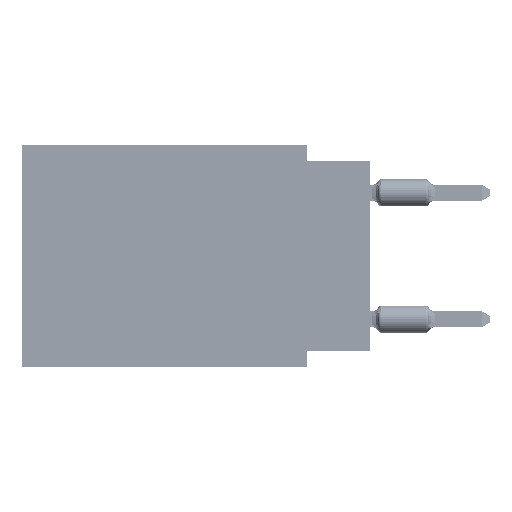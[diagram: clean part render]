
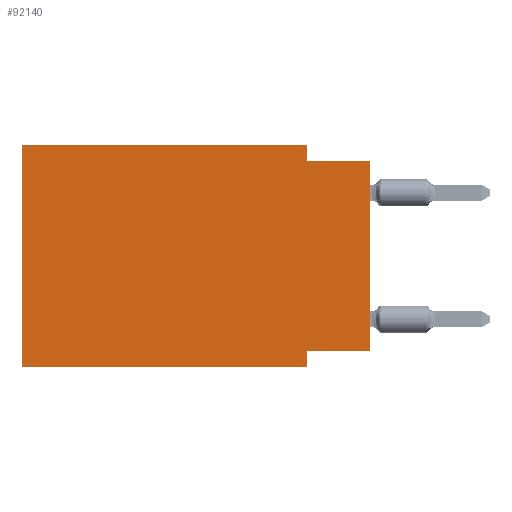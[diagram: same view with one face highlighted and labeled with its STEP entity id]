
A CAD part, left-side view. The second image highlights one B-rep face of the part: STEP entity #92140.
In plain terms, the highlighted planar face has unit normal (-1, 0, 0).
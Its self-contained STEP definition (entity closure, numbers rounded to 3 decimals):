
#493 = CARTESIAN_POINT ( 'NONE',  ( 0., 2.54, -8.89 ) ) ;
#1888 = CARTESIAN_POINT ( 'NONE',  ( 0., 13.97, 0. ) ) ;
#4435 = VECTOR ( 'NONE', #46885, 1000. ) ;
#5771 = VECTOR ( 'NONE', #45051, 1000. ) ;
#9405 = LINE ( 'NONE', #62555, #5771 ) ;
#11519 = CARTESIAN_POINT ( 'NONE',  ( 0., 0., -0.635 ) ) ;
#13031 = LINE ( 'NONE', #111192, #33113 ) ;
#13939 = VERTEX_POINT ( 'NONE', #55279 ) ;
#15241 = CARTESIAN_POINT ( 'NONE',  ( 0., 0., -0.635 ) ) ;
#15337 = FACE_OUTER_BOUND ( 'NONE', #18035, .T. ) ;
#15803 = LINE ( 'NONE', #51438, #30548 ) ;
#17249 = DIRECTION ( 'NONE',  ( 0., 0., -1. ) ) ;
#17670 = EDGE_CURVE ( 'NONE', #100016, #37350, #30232, .T. ) ;
#17733 = ORIENTED_EDGE ( 'NONE', *, *, #40142, .T. ) ;
#18035 = EDGE_LOOP ( 'NONE', ( #17733, #66285, #18633, #58168, #27498, #62420, #31094, #110468 ) ) ;
#18633 = ORIENTED_EDGE ( 'NONE', *, *, #108957, .F. ) ;
#22695 = VECTOR ( 'NONE', #17249, 1000. ) ;
#27498 = ORIENTED_EDGE ( 'NONE', *, *, #30764, .F. ) ;
#27574 = CARTESIAN_POINT ( 'NONE',  ( 0., 13.97, -8.89 ) ) ;
#29958 = CARTESIAN_POINT ( 'NONE',  ( 0., 2.54, -0.635 ) ) ;
#30232 = LINE ( 'NONE', #37839, #78064 ) ;
#30548 = VECTOR ( 'NONE', #78305, 1000. ) ;
#30764 = EDGE_CURVE ( 'NONE', #100016, #57945, #81920, .T. ) ;
#31094 = ORIENTED_EDGE ( 'NONE', *, *, #78271, .F. ) ;
#32855 = DIRECTION ( 'NONE',  ( 1., 0., 0. ) ) ;
#33113 = VECTOR ( 'NONE', #48692, 1000. ) ;
#35313 = VERTEX_POINT ( 'NONE', #29958 ) ;
#35346 = LINE ( 'NONE', #72120, #22695 ) ;
#37350 = VERTEX_POINT ( 'NONE', #493 ) ;
#37826 = DIRECTION ( 'NONE',  ( 0., 1., 0. ) ) ;
#37839 = CARTESIAN_POINT ( 'NONE',  ( 0., 13.97, -8.89 ) ) ;
#38108 = AXIS2_PLACEMENT_3D ( 'NONE', #61469, #32855, #42779 ) ;
#38359 = VERTEX_POINT ( 'NONE', #48074 ) ;
#40142 = EDGE_CURVE ( 'NONE', #38359, #90475, #13031, .T. ) ;
#41632 = PLANE ( 'NONE',  #38108 ) ;
#42779 = DIRECTION ( 'NONE',  ( 0., 0., -1. ) ) ;
#45051 = DIRECTION ( 'NONE',  ( 0., 0., -1. ) ) ;
#46885 = DIRECTION ( 'NONE',  ( 0., 0., 1. ) ) ;
#48074 = CARTESIAN_POINT ( 'NONE',  ( 0., 0., -8.255 ) ) ;
#48692 = DIRECTION ( 'NONE',  ( 0., 0., 1. ) ) ;
#51438 = CARTESIAN_POINT ( 'NONE',  ( 0., 13.97, 0. ) ) ;
#55279 = CARTESIAN_POINT ( 'NONE',  ( 0., 2.54, -8.255 ) ) ;
#55934 = DIRECTION ( 'NONE',  ( 0., -1., 0. ) ) ;
#56464 = EDGE_CURVE ( 'NONE', #57945, #102134, #15803, .T. ) ;
#57202 = CARTESIAN_POINT ( 'NONE',  ( 0., 13.97, 0. ) ) ;
#57323 = VECTOR ( 'NONE', #37826, 1000. ) ;
#57945 = VERTEX_POINT ( 'NONE', #57202 ) ;
#58168 = ORIENTED_EDGE ( 'NONE', *, *, #56464, .F. ) ;
#61469 = CARTESIAN_POINT ( 'NONE',  ( 0., 13.97, 0. ) ) ;
#62420 = ORIENTED_EDGE ( 'NONE', *, *, #17670, .T. ) ;
#62555 = CARTESIAN_POINT ( 'NONE',  ( 0., 2.54, -8.89 ) ) ;
#66285 = ORIENTED_EDGE ( 'NONE', *, *, #69022, .F. ) ;
#69022 = EDGE_CURVE ( 'NONE', #35313, #90475, #91560, .T. ) ;
#72120 = CARTESIAN_POINT ( 'NONE',  ( 0., 2.54, 0. ) ) ;
#73452 = CARTESIAN_POINT ( 'NONE',  ( 0., 0., -8.255 ) ) ;
#78064 = VECTOR ( 'NONE', #55934, 1000. ) ;
#78271 = EDGE_CURVE ( 'NONE', #13939, #37350, #9405, .T. ) ;
#78305 = DIRECTION ( 'NONE',  ( 0., -1., 0. ) ) ;
#81625 = LINE ( 'NONE', #73452, #57323 ) ;
#81920 = LINE ( 'NONE', #1888, #4435 ) ;
#82784 = DIRECTION ( 'NONE',  ( 0., -1., 0. ) ) ;
#90475 = VERTEX_POINT ( 'NONE', #15241 ) ;
#91560 = LINE ( 'NONE', #11519, #96959 ) ;
#92140 = ADVANCED_FACE ( 'NONE', ( #15337 ), #41632, .F. ) ;
#93863 = CARTESIAN_POINT ( 'NONE',  ( 0., 2.54, 0. ) ) ;
#96959 = VECTOR ( 'NONE', #82784, 1000. ) ;
#100016 = VERTEX_POINT ( 'NONE', #27574 ) ;
#102041 = EDGE_CURVE ( 'NONE', #38359, #13939, #81625, .T. ) ;
#102134 = VERTEX_POINT ( 'NONE', #93863 ) ;
#108957 = EDGE_CURVE ( 'NONE', #102134, #35313, #35346, .T. ) ;
#110468 = ORIENTED_EDGE ( 'NONE', *, *, #102041, .F. ) ;
#111192 = CARTESIAN_POINT ( 'NONE',  ( 0., 0., 0. ) ) ;
